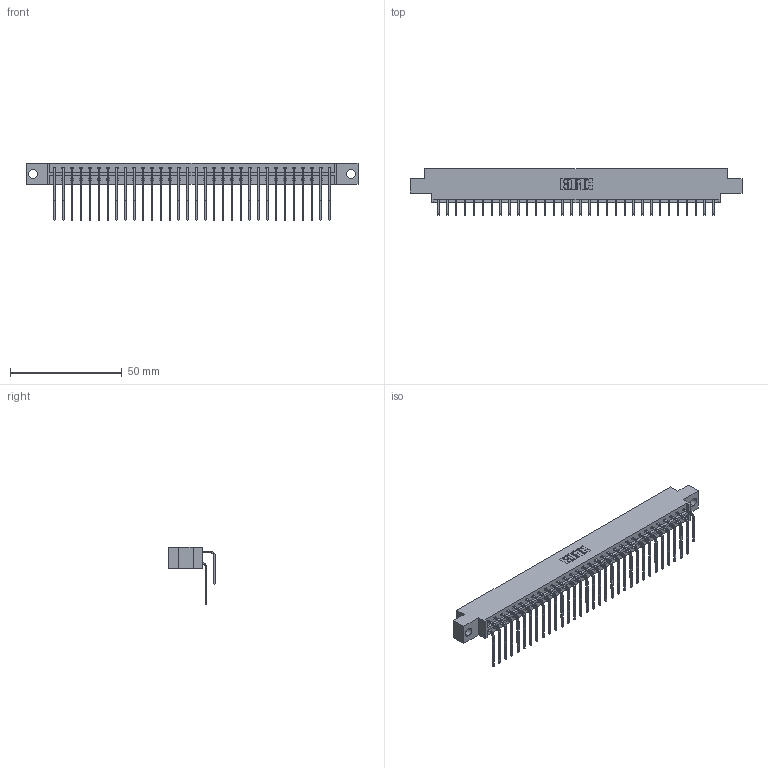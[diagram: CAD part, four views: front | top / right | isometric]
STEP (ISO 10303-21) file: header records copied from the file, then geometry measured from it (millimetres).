
FILE_DESCRIPTION (( 'STEP AP203' ), '1' );
FILE_NAME ('333-064-559-804.STEP', '2018-08-04T10:38:10', ( '' ), ( '' ), 'SwSTEP 2.0', 'SolidWorks 2016', '' );
FILE_SCHEMA (( 'CONFIG_CONTROL_DESIGN' ));
Length unit declared in the file: inch
Products named in the file (4): 333 Part_Offset - .156 Dia - TH; 345-292-001_558 559 Tail - 1; 345-292-001_559 Tail - 2; 333-064-559-804
Assembly tree (65 placements, depth 2):
  333-064-559-804
    333 Part_Offset - .156 Dia - TH
    345-292-001_558 559 Tail - 1  x32
    345-292-001_559 Tail - 2  x32
Bounding box: 148.34 x 20.9 x 25.53 mm (x, y, z)
Volume: 15104.3 mm3; surface area: 19608.8 mm2
Topology: 65 solids, 65 shells, 3574 faces, 10627 edges, 6998 vertices
Faces by surface type: plane 2506, cylinder 1068
Entity records: 23799 total; most frequent: CARTESIAN_POINT 4009, ORIENTED_EDGE 3894, DIRECTION 3423, EDGE_CURVE 1947, LINE 1779, VECTOR 1779, VERTEX_POINT 1294, AXIS2_PLACEMENT_3D 822
